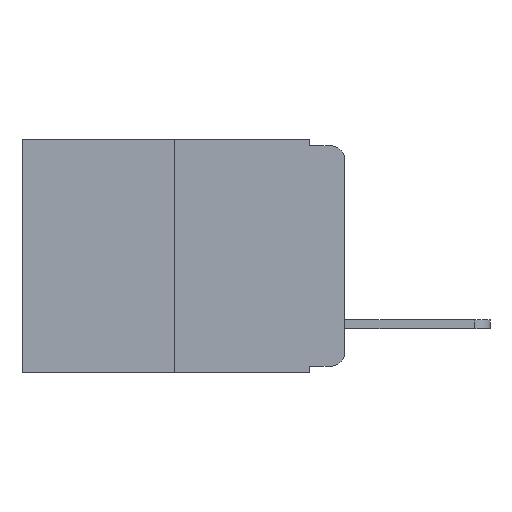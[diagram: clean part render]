
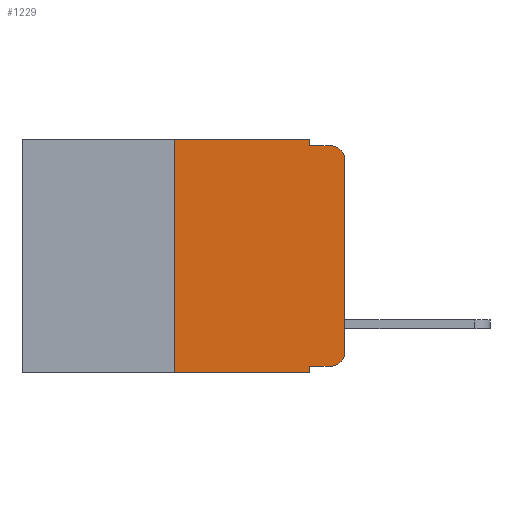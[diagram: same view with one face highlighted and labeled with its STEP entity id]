
A CAD part, left-side view. The second image highlights one B-rep face of the part: STEP entity #1229.
In plain terms, the highlighted planar face has unit normal (-1, 0, 0).
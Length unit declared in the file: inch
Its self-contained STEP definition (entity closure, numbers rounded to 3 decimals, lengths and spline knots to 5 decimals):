
#28 = CARTESIAN_POINT ( 'NONE',  ( 0., 0.25, -0.343 ) ) ;
#139 = CARTESIAN_POINT ( 'NONE',  ( 0., 0.02, -0.01 ) ) ;
#528 = VECTOR ( 'NONE', #5969, 39.37008 ) ;
#797 = DIRECTION ( 'NONE',  ( 0., 0., 1. ) ) ;
#813 = AXIS2_PLACEMENT_3D ( 'NONE', #9034, #10433, #3350 ) ;
#949 = DIRECTION ( 'NONE',  ( 1., 0., 0. ) ) ;
#1001 = CARTESIAN_POINT ( 'NONE',  ( 0., 0., -0.313 ) ) ;
#1123 = DIRECTION ( 'NONE',  ( 0., 0., -1. ) ) ;
#1229 = ADVANCED_FACE ( 'NONE', ( #8578 ), #7977, .F. ) ;
#2129 = VERTEX_POINT ( 'NONE', #11151 ) ;
#2340 = LINE ( 'NONE', #13451, #8264 ) ;
#2398 = LINE ( 'NONE', #5181, #8687 ) ;
#2568 = VERTEX_POINT ( 'NONE', #11425 ) ;
#2597 = DIRECTION ( 'NONE',  ( 0., 0., 1. ) ) ;
#2629 = VERTEX_POINT ( 'NONE', #28 ) ;
#2985 = DIRECTION ( 'NONE',  ( 0., -1., 0. ) ) ;
#3350 = DIRECTION ( 'NONE',  ( 0., 0., -1. ) ) ;
#3574 = VERTEX_POINT ( 'NONE', #1001 ) ;
#3945 = DIRECTION ( 'NONE',  ( 0., -1., 0. ) ) ;
#4249 = LINE ( 'NONE', #8854, #9731 ) ;
#4632 = EDGE_CURVE ( 'NONE', #6515, #3574, #5423, .T. ) ;
#4754 = DIRECTION ( 'NONE',  ( -1., 0., 0. ) ) ;
#5181 = CARTESIAN_POINT ( 'NONE',  ( 0., 0.051, 0. ) ) ;
#5423 = CIRCLE ( 'NONE', #813, 0.02 ) ;
#5428 = EDGE_CURVE ( 'NONE', #7636, #6515, #9930, .T. ) ;
#5969 = DIRECTION ( 'NONE',  ( 0., -1., 0. ) ) ;
#6156 = CARTESIAN_POINT ( 'NONE',  ( 0., 0.051, -0.01 ) ) ;
#6217 = EDGE_CURVE ( 'NONE', #7636, #10374, #2398, .T. ) ;
#6515 = VERTEX_POINT ( 'NONE', #12520 ) ;
#7025 = VECTOR ( 'NONE', #2597, 39.37008 ) ;
#7576 = LINE ( 'NONE', #6156, #13511 ) ;
#7636 = VERTEX_POINT ( 'NONE', #11039 ) ;
#7664 = ORIENTED_EDGE ( 'NONE', *, *, #4632, .T. ) ;
#7760 = ORIENTED_EDGE ( 'NONE', *, *, #5428, .T. ) ;
#7793 = EDGE_CURVE ( 'NONE', #2629, #14460, #2340, .T. ) ;
#7890 = CARTESIAN_POINT ( 'NONE',  ( 0., 0.473, 0. ) ) ;
#7977 = PLANE ( 'NONE',  #9340 ) ;
#8094 = ORIENTED_EDGE ( 'NONE', *, *, #9338, .F. ) ;
#8206 = VECTOR ( 'NONE', #10637, 39.37008 ) ;
#8264 = VECTOR ( 'NONE', #797, 39.37008 ) ;
#8407 = ORIENTED_EDGE ( 'NONE', *, *, #7793, .F. ) ;
#8430 = CIRCLE ( 'NONE', #12820, 0.02 ) ;
#8572 = ORIENTED_EDGE ( 'NONE', *, *, #9957, .T. ) ;
#8578 = FACE_OUTER_BOUND ( 'NONE', #11764, .T. ) ;
#8687 = VECTOR ( 'NONE', #13097, 39.37008 ) ;
#8839 = ORIENTED_EDGE ( 'NONE', *, *, #10828, .F. ) ;
#8854 = CARTESIAN_POINT ( 'NONE',  ( 0., 0.473, 0. ) ) ;
#9034 = CARTESIAN_POINT ( 'NONE',  ( 0., 0.02, -0.313 ) ) ;
#9262 = ORIENTED_EDGE ( 'NONE', *, *, #14493, .T. ) ;
#9338 = EDGE_CURVE ( 'NONE', #2568, #10352, #11181, .T. ) ;
#9340 = AXIS2_PLACEMENT_3D ( 'NONE', #7890, #949, #1123 ) ;
#9731 = VECTOR ( 'NONE', #2985, 39.37008 ) ;
#9806 = CARTESIAN_POINT ( 'NONE',  ( 0., 0.473, -0.343 ) ) ;
#9930 = LINE ( 'NONE', #13840, #528 ) ;
#9957 = EDGE_CURVE ( 'NONE', #2629, #10374, #11328, .T. ) ;
#10352 = VERTEX_POINT ( 'NONE', #13113 ) ;
#10374 = VERTEX_POINT ( 'NONE', #14271 ) ;
#10433 = DIRECTION ( 'NONE',  ( -1., 0., 0. ) ) ;
#10622 = CARTESIAN_POINT ( 'NONE',  ( 0., 0.25, 0. ) ) ;
#10637 = DIRECTION ( 'NONE',  ( 0., 0., -1. ) ) ;
#10709 = DIRECTION ( 'NONE',  ( 0., -1., 0. ) ) ;
#10828 = EDGE_CURVE ( 'NONE', #10352, #11961, #7576, .T. ) ;
#11039 = CARTESIAN_POINT ( 'NONE',  ( 0., 0.051, -0.333 ) ) ;
#11151 = CARTESIAN_POINT ( 'NONE',  ( 0., 0., -0.03 ) ) ;
#11181 = LINE ( 'NONE', #11789, #8206 ) ;
#11328 = LINE ( 'NONE', #9806, #13887 ) ;
#11425 = CARTESIAN_POINT ( 'NONE',  ( 0., 0.051, 0. ) ) ;
#11517 = EDGE_CURVE ( 'NONE', #14460, #2568, #4249, .T. ) ;
#11611 = CARTESIAN_POINT ( 'NONE',  ( 0., 0.02, -0.03 ) ) ;
#11764 = EDGE_LOOP ( 'NONE', ( #9262, #14169, #8839, #8094, #11905, #8407, #8572, #13447, #7760, #7664 ) ) ;
#11776 = CARTESIAN_POINT ( 'NONE',  ( 0., 0., 0. ) ) ;
#11789 = CARTESIAN_POINT ( 'NONE',  ( 0., 0.051, 0. ) ) ;
#11905 = ORIENTED_EDGE ( 'NONE', *, *, #11517, .F. ) ;
#11961 = VERTEX_POINT ( 'NONE', #139 ) ;
#12520 = CARTESIAN_POINT ( 'NONE',  ( 0., 0.02, -0.333 ) ) ;
#12704 = DIRECTION ( 'NONE',  ( 0., 0., -1. ) ) ;
#12820 = AXIS2_PLACEMENT_3D ( 'NONE', #11611, #4754, #12704 ) ;
#12998 = LINE ( 'NONE', #11776, #7025 ) ;
#13020 = EDGE_CURVE ( 'NONE', #2129, #11961, #8430, .T. ) ;
#13097 = DIRECTION ( 'NONE',  ( 0., 0., -1. ) ) ;
#13113 = CARTESIAN_POINT ( 'NONE',  ( 0., 0.051, -0.01 ) ) ;
#13447 = ORIENTED_EDGE ( 'NONE', *, *, #6217, .F. ) ;
#13451 = CARTESIAN_POINT ( 'NONE',  ( 0., 0.25, 0. ) ) ;
#13511 = VECTOR ( 'NONE', #10709, 39.37008 ) ;
#13840 = CARTESIAN_POINT ( 'NONE',  ( 0., 0.051, -0.333 ) ) ;
#13887 = VECTOR ( 'NONE', #3945, 39.37008 ) ;
#14169 = ORIENTED_EDGE ( 'NONE', *, *, #13020, .T. ) ;
#14271 = CARTESIAN_POINT ( 'NONE',  ( 0., 0.051, -0.343 ) ) ;
#14460 = VERTEX_POINT ( 'NONE', #10622 ) ;
#14493 = EDGE_CURVE ( 'NONE', #3574, #2129, #12998, .T. ) ;
